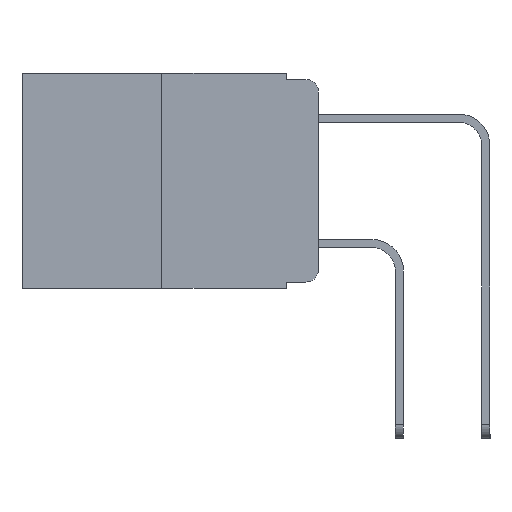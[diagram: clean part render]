
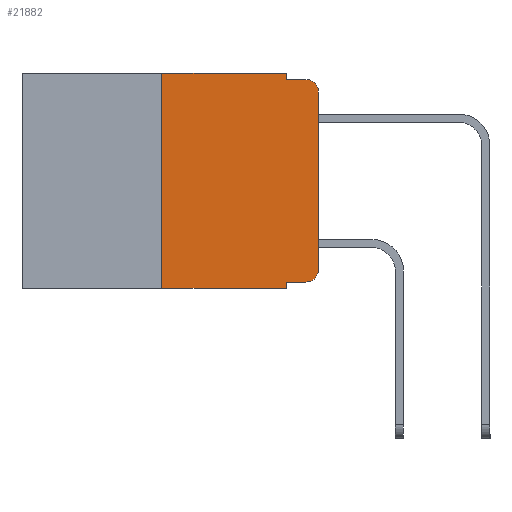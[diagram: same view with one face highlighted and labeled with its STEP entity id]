
A CAD part, left-side view. The second image highlights one B-rep face of the part: STEP entity #21882.
In plain terms, the highlighted planar face has unit normal (-1, 0, 0).
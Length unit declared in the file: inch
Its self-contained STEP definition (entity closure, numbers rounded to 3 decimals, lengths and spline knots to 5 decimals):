
#367 = CARTESIAN_POINT ( 'NONE',  ( 0., 0.25, 0. ) ) ;
#391 = AXIS2_PLACEMENT_3D ( 'NONE', #12776, #14801, #2500 ) ;
#1134 = LINE ( 'NONE', #16627, #18095 ) ;
#1275 = DIRECTION ( 'NONE',  ( 0., -1., 0. ) ) ;
#2018 = CIRCLE ( 'NONE', #23022, 0.02 ) ;
#2088 = VERTEX_POINT ( 'NONE', #7743 ) ;
#2107 = VERTEX_POINT ( 'NONE', #11870 ) ;
#2265 = CARTESIAN_POINT ( 'NONE',  ( 0., 0.051, -0.01 ) ) ;
#2408 = VECTOR ( 'NONE', #15669, 39.37008 ) ;
#2500 = DIRECTION ( 'NONE',  ( 0., 0., -1. ) ) ;
#2548 = ORIENTED_EDGE ( 'NONE', *, *, #4174, .F. ) ;
#2676 = EDGE_CURVE ( 'NONE', #5656, #2088, #15997, .T. ) ;
#3357 = VERTEX_POINT ( 'NONE', #15691 ) ;
#3668 = ORIENTED_EDGE ( 'NONE', *, *, #10280, .T. ) ;
#3721 = EDGE_CURVE ( 'NONE', #13708, #2107, #13452, .T. ) ;
#3779 = DIRECTION ( 'NONE',  ( 0., -1., 0. ) ) ;
#4174 = EDGE_CURVE ( 'NONE', #4417, #14667, #24008, .T. ) ;
#4417 = VERTEX_POINT ( 'NONE', #367 ) ;
#5181 = DIRECTION ( 'NONE',  ( -1., 0., 0. ) ) ;
#5613 = EDGE_CURVE ( 'NONE', #14667, #13708, #18050, .T. ) ;
#5656 = VERTEX_POINT ( 'NONE', #9731 ) ;
#5863 = DIRECTION ( 'NONE',  ( -1., 0., 0. ) ) ;
#6761 = ORIENTED_EDGE ( 'NONE', *, *, #18225, .F. ) ;
#6844 = EDGE_CURVE ( 'NONE', #2088, #22750, #17658, .T. ) ;
#7499 = CARTESIAN_POINT ( 'NONE',  ( 0., 0.473, -0.343 ) ) ;
#7743 = CARTESIAN_POINT ( 'NONE',  ( 0., 0.02, -0.333 ) ) ;
#7994 = VECTOR ( 'NONE', #3779, 39.37008 ) ;
#8017 = VECTOR ( 'NONE', #22661, 39.37008 ) ;
#8308 = VERTEX_POINT ( 'NONE', #22046 ) ;
#9594 = ORIENTED_EDGE ( 'NONE', *, *, #3721, .F. ) ;
#9650 = ORIENTED_EDGE ( 'NONE', *, *, #19565, .T. ) ;
#9731 = CARTESIAN_POINT ( 'NONE',  ( 0., 0.051, -0.333 ) ) ;
#10068 = CARTESIAN_POINT ( 'NONE',  ( 0., 0.051, 0. ) ) ;
#10102 = VECTOR ( 'NONE', #22106, 39.37008 ) ;
#10127 = EDGE_LOOP ( 'NONE', ( #14706, #3668, #9594, #12470, #2548, #6761, #9650, #12960, #12676, #11845 ) ) ;
#10280 = EDGE_CURVE ( 'NONE', #8308, #2107, #2018, .T. ) ;
#10633 = EDGE_CURVE ( 'NONE', #5656, #3357, #15497, .T. ) ;
#10651 = CARTESIAN_POINT ( 'NONE',  ( 0., 0.051, -0.01 ) ) ;
#10723 = PLANE ( 'NONE',  #391 ) ;
#11580 = CARTESIAN_POINT ( 'NONE',  ( 0., 0.051, -0.333 ) ) ;
#11845 = ORIENTED_EDGE ( 'NONE', *, *, #6844, .T. ) ;
#11870 = CARTESIAN_POINT ( 'NONE',  ( 0., 0.02, -0.01 ) ) ;
#11954 = CARTESIAN_POINT ( 'NONE',  ( 0., 0.473, 0. ) ) ;
#12470 = ORIENTED_EDGE ( 'NONE', *, *, #5613, .F. ) ;
#12676 = ORIENTED_EDGE ( 'NONE', *, *, #2676, .T. ) ;
#12776 = CARTESIAN_POINT ( 'NONE',  ( 0., 0.473, 0. ) ) ;
#12851 = DIRECTION ( 'NONE',  ( 0., 0., 1. ) ) ;
#12960 = ORIENTED_EDGE ( 'NONE', *, *, #10633, .F. ) ;
#13452 = LINE ( 'NONE', #10651, #8017 ) ;
#13682 = FACE_OUTER_BOUND ( 'NONE', #10127, .T. ) ;
#13708 = VERTEX_POINT ( 'NONE', #2265 ) ;
#13774 = AXIS2_PLACEMENT_3D ( 'NONE', #17358, #5181, #19369 ) ;
#13943 = LINE ( 'NONE', #7499, #18656 ) ;
#14206 = CARTESIAN_POINT ( 'NONE',  ( 0., 0.25, -0.343 ) ) ;
#14667 = VERTEX_POINT ( 'NONE', #23825 ) ;
#14706 = ORIENTED_EDGE ( 'NONE', *, *, #25002, .T. ) ;
#14801 = DIRECTION ( 'NONE',  ( 1., 0., 0. ) ) ;
#15497 = LINE ( 'NONE', #10068, #10102 ) ;
#15669 = DIRECTION ( 'NONE',  ( 0., 0., -1. ) ) ;
#15691 = CARTESIAN_POINT ( 'NONE',  ( 0., 0.051, -0.343 ) ) ;
#15997 = LINE ( 'NONE', #11580, #25906 ) ;
#16320 = LINE ( 'NONE', #16412, #26210 ) ;
#16412 = CARTESIAN_POINT ( 'NONE',  ( 0., 0., 0. ) ) ;
#16627 = CARTESIAN_POINT ( 'NONE',  ( 0., 0.25, 0. ) ) ;
#17358 = CARTESIAN_POINT ( 'NONE',  ( 0., 0.02, -0.313 ) ) ;
#17658 = CIRCLE ( 'NONE', #13774, 0.02 ) ;
#18032 = CARTESIAN_POINT ( 'NONE',  ( 0., 0.02, -0.03 ) ) ;
#18050 = LINE ( 'NONE', #25195, #2408 ) ;
#18095 = VECTOR ( 'NONE', #24517, 39.37008 ) ;
#18225 = EDGE_CURVE ( 'NONE', #19374, #4417, #1134, .T. ) ;
#18656 = VECTOR ( 'NONE', #19625, 39.37008 ) ;
#19369 = DIRECTION ( 'NONE',  ( 0., 0., -1. ) ) ;
#19374 = VERTEX_POINT ( 'NONE', #14206 ) ;
#19565 = EDGE_CURVE ( 'NONE', #19374, #3357, #13943, .T. ) ;
#19625 = DIRECTION ( 'NONE',  ( 0., -1., 0. ) ) ;
#20051 = DIRECTION ( 'NONE',  ( 0., 0., -1. ) ) ;
#21882 = ADVANCED_FACE ( 'NONE', ( #13682 ), #10723, .F. ) ;
#22046 = CARTESIAN_POINT ( 'NONE',  ( 0., 0., -0.03 ) ) ;
#22106 = DIRECTION ( 'NONE',  ( 0., 0., -1. ) ) ;
#22661 = DIRECTION ( 'NONE',  ( 0., -1., 0. ) ) ;
#22750 = VERTEX_POINT ( 'NONE', #23320 ) ;
#23022 = AXIS2_PLACEMENT_3D ( 'NONE', #18032, #5863, #20051 ) ;
#23320 = CARTESIAN_POINT ( 'NONE',  ( 0., 0., -0.313 ) ) ;
#23825 = CARTESIAN_POINT ( 'NONE',  ( 0., 0.051, 0. ) ) ;
#24008 = LINE ( 'NONE', #11954, #7994 ) ;
#24517 = DIRECTION ( 'NONE',  ( 0., 0., 1. ) ) ;
#25002 = EDGE_CURVE ( 'NONE', #22750, #8308, #16320, .T. ) ;
#25195 = CARTESIAN_POINT ( 'NONE',  ( 0., 0.051, 0. ) ) ;
#25906 = VECTOR ( 'NONE', #1275, 39.37008 ) ;
#26210 = VECTOR ( 'NONE', #12851, 39.37008 ) ;
